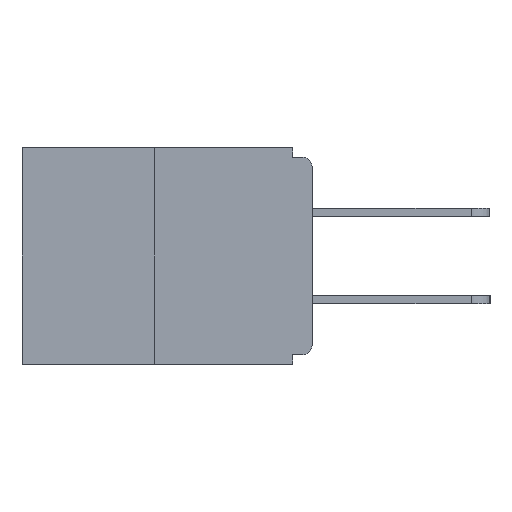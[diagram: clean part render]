
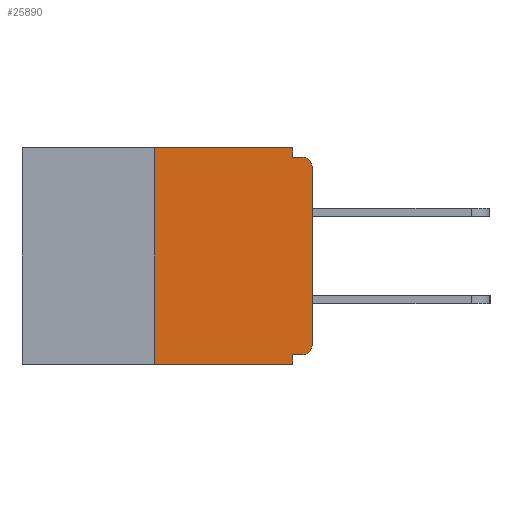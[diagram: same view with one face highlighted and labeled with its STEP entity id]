
A CAD part, left-side view. The second image highlights one B-rep face of the part: STEP entity #25890.
In plain terms, the highlighted planar face has unit normal (-1, 0, 0).
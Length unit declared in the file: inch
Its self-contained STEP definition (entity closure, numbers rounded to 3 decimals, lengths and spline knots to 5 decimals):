
#180 = CARTESIAN_POINT ( 'NONE',  ( 0., 0.015, -0.328 ) ) ;
#696 = VECTOR ( 'NONE', #26661, 39.37008 ) ;
#884 = EDGE_CURVE ( 'NONE', #17919, #10401, #7886, .T. ) ;
#948 = CIRCLE ( 'NONE', #18628, 0.015 ) ;
#1046 = CARTESIAN_POINT ( 'NONE',  ( 0., 0.25, 0. ) ) ;
#1099 = VECTOR ( 'NONE', #20522, 39.37008 ) ;
#1341 = CARTESIAN_POINT ( 'NONE',  ( 0., 0., -0.03 ) ) ;
#1807 = DIRECTION ( 'NONE',  ( 0., 0., -1. ) ) ;
#1922 = EDGE_CURVE ( 'NONE', #4813, #8470, #948, .T. ) ;
#2184 = LINE ( 'NONE', #19191, #12720 ) ;
#2774 = DIRECTION ( 'NONE',  ( -1., 0., 0. ) ) ;
#3052 = CARTESIAN_POINT ( 'NONE',  ( 0., 0.031, -0.343 ) ) ;
#3887 = ORIENTED_EDGE ( 'NONE', *, *, #19746, .F. ) ;
#3959 = DIRECTION ( 'NONE',  ( 0., 0., -1. ) ) ;
#3990 = CARTESIAN_POINT ( 'NONE',  ( 0., 0.25, -0.343 ) ) ;
#4016 = CARTESIAN_POINT ( 'NONE',  ( 0., 0., 0. ) ) ;
#4169 = CARTESIAN_POINT ( 'NONE',  ( 0., 0., -0.328 ) ) ;
#4263 = FACE_OUTER_BOUND ( 'NONE', #19497, .T. ) ;
#4813 = VERTEX_POINT ( 'NONE', #1341 ) ;
#5114 = DIRECTION ( 'NONE',  ( 0., -1., 0. ) ) ;
#6361 = VECTOR ( 'NONE', #1807, 39.37008 ) ;
#6379 = CIRCLE ( 'NONE', #21494, 0.015 ) ;
#6800 = CARTESIAN_POINT ( 'NONE',  ( 0., 0.015, -0.015 ) ) ;
#7705 = CARTESIAN_POINT ( 'NONE',  ( 0., 0., -0.313 ) ) ;
#7886 = LINE ( 'NONE', #22895, #21159 ) ;
#8192 = PLANE ( 'NONE',  #14466 ) ;
#8470 = VERTEX_POINT ( 'NONE', #6800 ) ;
#8723 = CARTESIAN_POINT ( 'NONE',  ( 0., 0.46, 0. ) ) ;
#9197 = ORIENTED_EDGE ( 'NONE', *, *, #24313, .F. ) ;
#9592 = ORIENTED_EDGE ( 'NONE', *, *, #17556, .F. ) ;
#10326 = CARTESIAN_POINT ( 'NONE',  ( 0., 0.031, -0.015 ) ) ;
#10368 = LINE ( 'NONE', #22529, #19963 ) ;
#10401 = VERTEX_POINT ( 'NONE', #14259 ) ;
#10579 = EDGE_CURVE ( 'NONE', #15104, #22732, #10368, .T. ) ;
#11087 = EDGE_CURVE ( 'NONE', #17248, #11928, #6379, .T. ) ;
#11928 = VERTEX_POINT ( 'NONE', #7705 ) ;
#11956 = CARTESIAN_POINT ( 'NONE',  ( 0., 0.015, -0.313 ) ) ;
#12282 = CARTESIAN_POINT ( 'NONE',  ( 0., 0.031, -0.328 ) ) ;
#12293 = VECTOR ( 'NONE', #5114, 39.37008 ) ;
#12720 = VECTOR ( 'NONE', #25306, 39.37008 ) ;
#13909 = DIRECTION ( 'NONE',  ( 0., 0., 1. ) ) ;
#14259 = CARTESIAN_POINT ( 'NONE',  ( 0., 0.031, 0. ) ) ;
#14466 = AXIS2_PLACEMENT_3D ( 'NONE', #8723, #14542, #14801 ) ;
#14542 = DIRECTION ( 'NONE',  ( 1., 0., 0. ) ) ;
#14801 = DIRECTION ( 'NONE',  ( 0., 0., -1. ) ) ;
#15088 = DIRECTION ( 'NONE',  ( 0., 0., -1. ) ) ;
#15097 = CARTESIAN_POINT ( 'NONE',  ( 0., 0., -0.015 ) ) ;
#15098 = ORIENTED_EDGE ( 'NONE', *, *, #1922, .T. ) ;
#15104 = VERTEX_POINT ( 'NONE', #12282 ) ;
#16040 = VERTEX_POINT ( 'NONE', #10326 ) ;
#16969 = ORIENTED_EDGE ( 'NONE', *, *, #25253, .T. ) ;
#17116 = LINE ( 'NONE', #15097, #696 ) ;
#17248 = VERTEX_POINT ( 'NONE', #180 ) ;
#17405 = LINE ( 'NONE', #19702, #12293 ) ;
#17556 = EDGE_CURVE ( 'NONE', #17248, #15104, #18217, .T. ) ;
#17919 = VERTEX_POINT ( 'NONE', #1046 ) ;
#18005 = VERTEX_POINT ( 'NONE', #3990 ) ;
#18217 = LINE ( 'NONE', #4169, #1099 ) ;
#18292 = ORIENTED_EDGE ( 'NONE', *, *, #23232, .F. ) ;
#18460 = DIRECTION ( 'NONE',  ( 0., 0., -1. ) ) ;
#18628 = AXIS2_PLACEMENT_3D ( 'NONE', #21433, #2774, #15088 ) ;
#19191 = CARTESIAN_POINT ( 'NONE',  ( 0., 0.25, 0. ) ) ;
#19497 = EDGE_LOOP ( 'NONE', ( #24939, #18292, #23131, #23517, #9592, #21804, #16969, #15098, #9197, #3887 ) ) ;
#19702 = CARTESIAN_POINT ( 'NONE',  ( 0., 0.46, -0.343 ) ) ;
#19746 = EDGE_CURVE ( 'NONE', #10401, #16040, #20333, .T. ) ;
#19963 = VECTOR ( 'NONE', #18460, 39.37008 ) ;
#20198 = DIRECTION ( 'NONE',  ( -1., 0., 0. ) ) ;
#20333 = LINE ( 'NONE', #21972, #6361 ) ;
#20380 = LINE ( 'NONE', #4016, #20935 ) ;
#20522 = DIRECTION ( 'NONE',  ( 0., 1., 0. ) ) ;
#20935 = VECTOR ( 'NONE', #13909, 39.37008 ) ;
#21159 = VECTOR ( 'NONE', #24931, 39.37008 ) ;
#21433 = CARTESIAN_POINT ( 'NONE',  ( 0., 0.015, -0.03 ) ) ;
#21494 = AXIS2_PLACEMENT_3D ( 'NONE', #11956, #20198, #3959 ) ;
#21804 = ORIENTED_EDGE ( 'NONE', *, *, #11087, .T. ) ;
#21972 = CARTESIAN_POINT ( 'NONE',  ( 0., 0.031, 0. ) ) ;
#22529 = CARTESIAN_POINT ( 'NONE',  ( 0., 0.031, -0.343 ) ) ;
#22732 = VERTEX_POINT ( 'NONE', #3052 ) ;
#22895 = CARTESIAN_POINT ( 'NONE',  ( 0., 0.46, 0. ) ) ;
#23131 = ORIENTED_EDGE ( 'NONE', *, *, #23901, .T. ) ;
#23232 = EDGE_CURVE ( 'NONE', #18005, #17919, #2184, .T. ) ;
#23517 = ORIENTED_EDGE ( 'NONE', *, *, #10579, .F. ) ;
#23901 = EDGE_CURVE ( 'NONE', #18005, #22732, #17405, .T. ) ;
#24313 = EDGE_CURVE ( 'NONE', #16040, #8470, #17116, .T. ) ;
#24931 = DIRECTION ( 'NONE',  ( 0., -1., 0. ) ) ;
#24939 = ORIENTED_EDGE ( 'NONE', *, *, #884, .F. ) ;
#25253 = EDGE_CURVE ( 'NONE', #11928, #4813, #20380, .T. ) ;
#25306 = DIRECTION ( 'NONE',  ( 0., 0., 1. ) ) ;
#25890 = ADVANCED_FACE ( 'NONE', ( #4263 ), #8192, .F. ) ;
#26661 = DIRECTION ( 'NONE',  ( 0., -1., 0. ) ) ;
